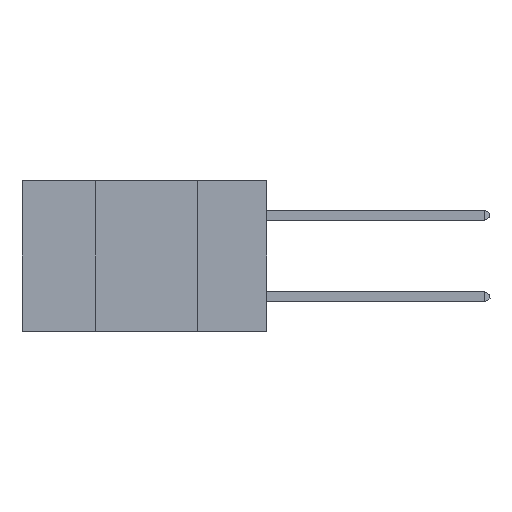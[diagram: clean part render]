
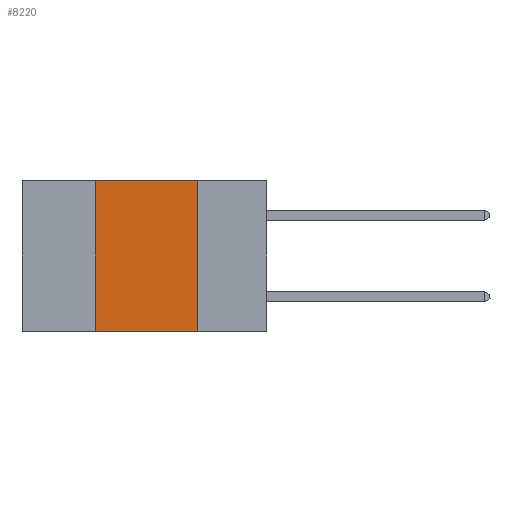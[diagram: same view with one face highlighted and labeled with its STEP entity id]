
A CAD part, left-side view. The second image highlights one B-rep face of the part: STEP entity #8220.
In plain terms, the highlighted planar face has unit normal (-1, 0, 0).
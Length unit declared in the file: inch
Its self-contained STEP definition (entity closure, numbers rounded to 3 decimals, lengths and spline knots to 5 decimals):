
#273 = DIRECTION ( 'NONE',  ( 1., 0., 0. ) ) ;
#787 = DIRECTION ( 'NONE',  ( 0., 0., -1. ) ) ;
#2268 = VECTOR ( 'NONE', #13648, 39.37008 ) ;
#3104 = CARTESIAN_POINT ( 'NONE',  ( 0., 0.6, 0. ) ) ;
#3378 = EDGE_CURVE ( 'NONE', #18278, #4734, #9723, .T. ) ;
#3421 = ORIENTED_EDGE ( 'NONE', *, *, #5429, .F. ) ;
#3460 = ORIENTED_EDGE ( 'NONE', *, *, #18166, .F. ) ;
#3601 = VERTEX_POINT ( 'NONE', #7107 ) ;
#3702 = CARTESIAN_POINT ( 'NONE',  ( 0., 0.17, -0.37 ) ) ;
#3892 = VECTOR ( 'NONE', #17114, 39.37008 ) ;
#4734 = VERTEX_POINT ( 'NONE', #6833 ) ;
#5429 = EDGE_CURVE ( 'NONE', #3601, #15132, #17142, .T. ) ;
#5456 = ORIENTED_EDGE ( 'NONE', *, *, #3378, .F. ) ;
#5815 = ORIENTED_EDGE ( 'NONE', *, *, #10253, .T. ) ;
#6046 = VECTOR ( 'NONE', #787, 39.37008 ) ;
#6486 = CARTESIAN_POINT ( 'NONE',  ( 0., 0.6, 0. ) ) ;
#6833 = CARTESIAN_POINT ( 'NONE',  ( 0., 0.42, 0. ) ) ;
#6926 = LINE ( 'NONE', #10296, #3892 ) ;
#7107 = CARTESIAN_POINT ( 'NONE',  ( 0., 0.17, 0. ) ) ;
#7668 = FACE_OUTER_BOUND ( 'NONE', #16578, .T. ) ;
#8220 = ADVANCED_FACE ( 'NONE', ( #7668 ), #9370, .F. ) ;
#9370 = PLANE ( 'NONE',  #17150 ) ;
#9723 = LINE ( 'NONE', #17786, #2268 ) ;
#10253 = EDGE_CURVE ( 'NONE', #18278, #15132, #6926, .T. ) ;
#10296 = CARTESIAN_POINT ( 'NONE',  ( 0., 0.6, -0.37 ) ) ;
#10758 = DIRECTION ( 'NONE',  ( 0., 0., -1. ) ) ;
#11365 = LINE ( 'NONE', #3104, #15440 ) ;
#11856 = CARTESIAN_POINT ( 'NONE',  ( 0., 0.42, -0.37 ) ) ;
#13648 = DIRECTION ( 'NONE',  ( 0., 0., 1. ) ) ;
#14547 = DIRECTION ( 'NONE',  ( 0., -1., 0. ) ) ;
#15132 = VERTEX_POINT ( 'NONE', #3702 ) ;
#15260 = CARTESIAN_POINT ( 'NONE',  ( 0., 0.17, 0. ) ) ;
#15440 = VECTOR ( 'NONE', #14547, 39.37008 ) ;
#16578 = EDGE_LOOP ( 'NONE', ( #3421, #3460, #5456, #5815 ) ) ;
#17114 = DIRECTION ( 'NONE',  ( 0., -1., 0. ) ) ;
#17142 = LINE ( 'NONE', #15260, #6046 ) ;
#17150 = AXIS2_PLACEMENT_3D ( 'NONE', #6486, #273, #10758 ) ;
#17786 = CARTESIAN_POINT ( 'NONE',  ( 0., 0.42, 0. ) ) ;
#18166 = EDGE_CURVE ( 'NONE', #4734, #3601, #11365, .T. ) ;
#18278 = VERTEX_POINT ( 'NONE', #11856 ) ;
